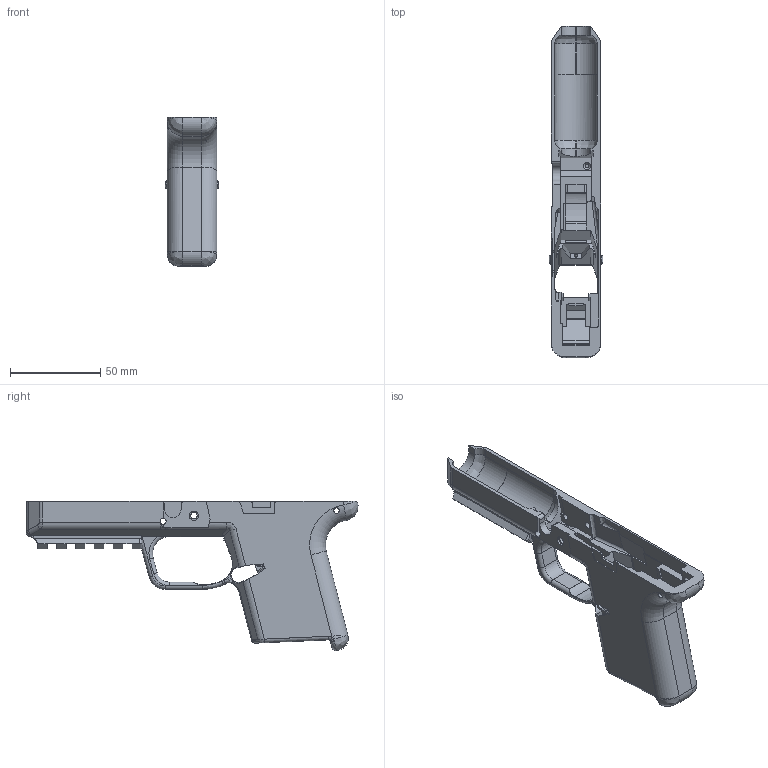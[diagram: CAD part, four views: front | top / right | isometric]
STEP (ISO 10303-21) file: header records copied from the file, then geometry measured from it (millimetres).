
FILE_DESCRIPTION(/* description */ (''),/* implementation_level */ '2;1');
FILE_NAME(/* name */ 'Girsan MC28SA - (M&P 9 Standard Length Slide - Picatinny).step',/* time_stamp */ '2022-02-23T00:58:01-05:00',/* author */ (''),/* organization */ (''),/* preprocessor_version */ 'ST-DEVELOPER v18.1',/* originating_system */ 'Autodesk Translation Framework v10.13.0.1454',/* authorisation */ '');
FILE_SCHEMA (('AUTOMOTIVE_DESIGN { 1 0 10303 214 3 1 1 }'));
Length unit declared in the file: millimetre
Products named in the file (6): Girsan MC28SA - (M&P 9 Standard Length Slide - Picatinny); M&P 9 Reference v116; Frame; Trigger Guard and Magwell; Fitment Section; M1.0 Full-size Nose
Assembly tree (5 placements, depth 5):
  Girsan MC28SA - (M&P 9 Standard Length Slide - Picatinny)
    M&P 9 Reference v116
      Frame
        Trigger Guard and Magwell
        Fitment Section
          M1.0 Full-size Nose
Bounding box: 29.75 x 183.61 x 82.48 mm (x, y, z)
Volume: 73690.1 mm3; surface area: 41104.2 mm2
Topology: 3 solids, 3 shells, 446 faces, 1228 edges, 774 vertices
Faces by surface type: plane 220, cylinder 134, bspline 69, torus 18, sphere 3, cone 2
Full cylindrical faces by diameter (mm): 1.5 x2, 3.18 x2, 3.361 x2, 3.55 x2, 5.1 x1
Entity records: 16310 total; most frequent: CARTESIAN_POINT 5017, ORIENTED_EDGE 2448, DIRECTION 2212, EDGE_CURVE 1224, VERTEX_POINT 774, LINE 746, VECTOR 746, AXIS2_PLACEMENT_3D 733
